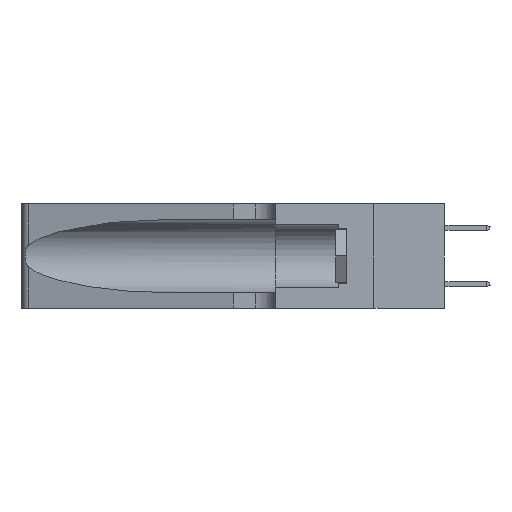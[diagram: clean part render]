
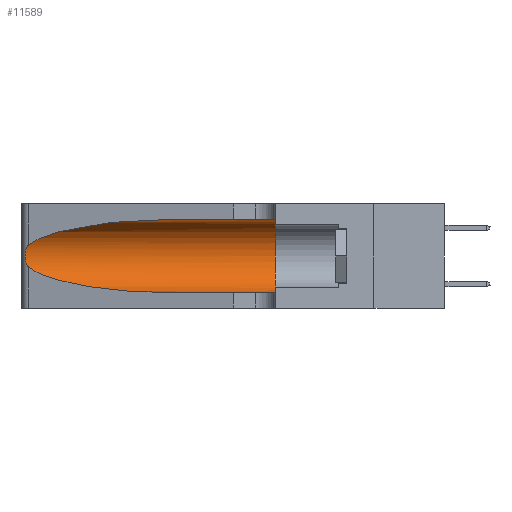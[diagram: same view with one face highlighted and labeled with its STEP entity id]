
A CAD part, left-side view. The second image highlights one B-rep face of the part: STEP entity #11589.
In plain terms, the highlighted cylindrical face has radius 3.308 mm (diameter 6.617 mm), a partial arc.
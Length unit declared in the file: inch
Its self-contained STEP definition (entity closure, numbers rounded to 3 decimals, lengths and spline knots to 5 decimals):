
#50 = CARTESIAN_POINT ( 'NONE',  ( 0.2373, 1.15595, 0.08982 ) ) ;
#750 = DIRECTION ( 'NONE',  ( 0., -1., 0. ) ) ;
#981 = CARTESIAN_POINT ( 'NONE',  ( 0.25487, 1.22718, 0.14631 ) ) ;
#1070 = CARTESIAN_POINT ( 'NONE',  ( 0.1305, 0.72297, 0.05475 ) ) ;
#1353 = ORIENTED_EDGE ( 'NONE', *, *, #11128, .T. ) ;
#1881 = CARTESIAN_POINT ( 'NONE',  ( 0.25854, 1.2359, 0.20912 ) ) ;
#2598 = DIRECTION ( 'NONE',  ( 0., 0., -1. ) ) ;
#2912 = CARTESIAN_POINT ( 'NONE',  ( 0.18966, 0.96281, 0.05475 ) ) ;
#3072 = CARTESIAN_POINT ( 'NONE',  ( 0.25487, 1.22718, 0.14631 ) ) ;
#3379 = CARTESIAN_POINT ( 'NONE',  ( 0.1305, 0.72297, 0.31525 ) ) ;
#3568 = CYLINDRICAL_SURFACE ( 'NONE', #12679, 0.13025 ) ;
#4127 = VECTOR ( 'NONE', #750, 39.37008 ) ;
#4443 = CARTESIAN_POINT ( 'NONE',  ( 0.25555, 1.22994, 0.2215 ) ) ;
#4525 = ORIENTED_EDGE ( 'NONE', *, *, #11468, .T. ) ;
#4550 = CARTESIAN_POINT ( 'NONE',  ( 0.26075, 1.23896, 0.178 ) ) ;
#4608 = FACE_OUTER_BOUND ( 'NONE', #9233, .T. ) ;
#4613 = EDGE_CURVE ( 'NONE', #14317, #5669, #8028, .T. ) ;
#4846 = CARTESIAN_POINT ( 'NONE',  ( 0.25555, 1.22993, 0.14849 ) ) ;
#5669 = VERTEX_POINT ( 'NONE', #1070 ) ;
#5777 = ORIENTED_EDGE ( 'NONE', *, *, #4613, .T. ) ;
#6099 = CARTESIAN_POINT ( 'NONE',  ( 0.25487, 1.22718, 0.22369 ) ) ;
#6118 = LINE ( 'NONE', #16669, #8692 ) ;
#6200 = VERTEX_POINT ( 'NONE', #15622 ) ;
#6214 = EDGE_CURVE ( 'NONE', #5669, #16711, #14365, .T. ) ;
#6279 = CARTESIAN_POINT ( 'NONE',  ( 0.25639, 1.23186, 0.15144 ) ) ;
#6796 = DIRECTION ( 'NONE',  ( 0., -1., 0. ) ) ;
#7279 = CARTESIAN_POINT ( 'NONE',  ( 0.26018, 1.23835, 0.19895 ) ) ;
#7296 = CIRCLE ( 'NONE', #17057, 0.13025 ) ;
#7587 = CARTESIAN_POINT ( 'NONE',  ( 0.25856, 1.23593, 0.16098 ) ) ;
#8028 =( BOUNDED_CURVE ( )  B_SPLINE_CURVE ( 3, ( #13803, #50, #2912, #9542 ),
 .UNSPECIFIED., .F., .F. ) 
 B_SPLINE_CURVE_WITH_KNOTS ( ( 4, 4 ),
 ( 3.44316, 4.71239 ),
 .UNSPECIFIED. ) 
 CURVE ( )  GEOMETRIC_REPRESENTATION_ITEM ( )  RATIONAL_B_SPLINE_CURVE ( ( 1., 0.87, 0.87, 1. ) ) 
 REPRESENTATION_ITEM ( '' )  );
#8118 = CARTESIAN_POINT ( 'NONE',  ( 0.1305, 0.35, 0.185 ) ) ;
#8186 = ORIENTED_EDGE ( 'NONE', *, *, #10033, .F. ) ;
#8692 = VECTOR ( 'NONE', #16484, 39.37008 ) ;
#8874 = B_SPLINE_CURVE_WITH_KNOTS ( 'NONE', 3,
 ( #16841, #4443, #15461, #10020, #1881, #7279, #14460, #4550, #14112, #7587, #12784, #6279, #4846, #3072 ),
 .UNSPECIFIED., .F., .F.,
 ( 4, 2, 2, 2, 2, 2, 4 ),
 ( 0., 0.00027, 0.00053, 0.00107, 0.0016, 0.00187, 0.00214 ),
 .UNSPECIFIED. ) ;
#9233 = EDGE_LOOP ( 'NONE', ( #1353, #4525, #5777, #11718, #11813, #8186 ) ) ;
#9542 = CARTESIAN_POINT ( 'NONE',  ( 0.1305, 0.72297, 0.05475 ) ) ;
#10020 = CARTESIAN_POINT ( 'NONE',  ( 0.25787, 1.23484, 0.2124 ) ) ;
#10033 = EDGE_CURVE ( 'NONE', #10945, #13243, #6118, .T. ) ;
#10315 = CARTESIAN_POINT ( 'NONE',  ( 0.2373, 1.15595, 0.28018 ) ) ;
#10595 = CARTESIAN_POINT ( 'NONE',  ( 0.1305, 0.72297, 0.31525 ) ) ;
#10945 = VERTEX_POINT ( 'NONE', #10595 ) ;
#11128 = EDGE_CURVE ( 'NONE', #10945, #6200, #16011, .T. ) ;
#11468 = EDGE_CURVE ( 'NONE', #6200, #14317, #8874, .T. ) ;
#11589 = ADVANCED_FACE ( 'NONE', ( #4608 ), #3568, .F. ) ;
#11718 = ORIENTED_EDGE ( 'NONE', *, *, #6214, .T. ) ;
#11813 = ORIENTED_EDGE ( 'NONE', *, *, #13709, .F. ) ;
#12243 = CARTESIAN_POINT ( 'NONE',  ( 0.1305, 1.61858, 0.185 ) ) ;
#12679 = AXIS2_PLACEMENT_3D ( 'NONE', #12243, #6796, #2598 ) ;
#12784 = CARTESIAN_POINT ( 'NONE',  ( 0.25789, 1.23486, 0.15765 ) ) ;
#13243 = VERTEX_POINT ( 'NONE', #14939 ) ;
#13390 = DIRECTION ( 'NONE',  ( 0., 1., 0. ) ) ;
#13709 = EDGE_CURVE ( 'NONE', #13243, #16711, #7296, .T. ) ;
#13803 = CARTESIAN_POINT ( 'NONE',  ( 0.25487, 1.22718, 0.14631 ) ) ;
#13887 = CARTESIAN_POINT ( 'NONE',  ( 0.1305, 0.35, 0.05475 ) ) ;
#14112 = CARTESIAN_POINT ( 'NONE',  ( 0.26017, 1.23833, 0.17102 ) ) ;
#14282 = CARTESIAN_POINT ( 'NONE',  ( 0.18966, 0.96281, 0.31525 ) ) ;
#14317 = VERTEX_POINT ( 'NONE', #981 ) ;
#14365 = LINE ( 'NONE', #17075, #4127 ) ;
#14460 = CARTESIAN_POINT ( 'NONE',  ( 0.26075, 1.23896, 0.19203 ) ) ;
#14939 = CARTESIAN_POINT ( 'NONE',  ( 0.1305, 0.35, 0.31525 ) ) ;
#15461 = CARTESIAN_POINT ( 'NONE',  ( 0.25639, 1.23184, 0.21858 ) ) ;
#15622 = CARTESIAN_POINT ( 'NONE',  ( 0.25487, 1.22718, 0.22369 ) ) ;
#16011 =( BOUNDED_CURVE ( )  B_SPLINE_CURVE ( 3, ( #3379, #14282, #10315, #6099 ),
 .UNSPECIFIED., .F., .F. ) 
 B_SPLINE_CURVE_WITH_KNOTS ( ( 4, 4 ),
 ( 1.5708, 2.84003 ),
 .UNSPECIFIED. ) 
 CURVE ( )  GEOMETRIC_REPRESENTATION_ITEM ( )  RATIONAL_B_SPLINE_CURVE ( ( 1., 0.87, 0.87, 1. ) ) 
 REPRESENTATION_ITEM ( '' )  );
#16352 = DIRECTION ( 'NONE',  ( 0., 0., 1. ) ) ;
#16484 = DIRECTION ( 'NONE',  ( 0., -1., 0. ) ) ;
#16669 = CARTESIAN_POINT ( 'NONE',  ( 0.1305, 1.61858, 0.31525 ) ) ;
#16711 = VERTEX_POINT ( 'NONE', #13887 ) ;
#16841 = CARTESIAN_POINT ( 'NONE',  ( 0.25487, 1.22718, 0.22369 ) ) ;
#17057 = AXIS2_PLACEMENT_3D ( 'NONE', #8118, #13390, #16352 ) ;
#17075 = CARTESIAN_POINT ( 'NONE',  ( 0.1305, 1.61858, 0.05475 ) ) ;
